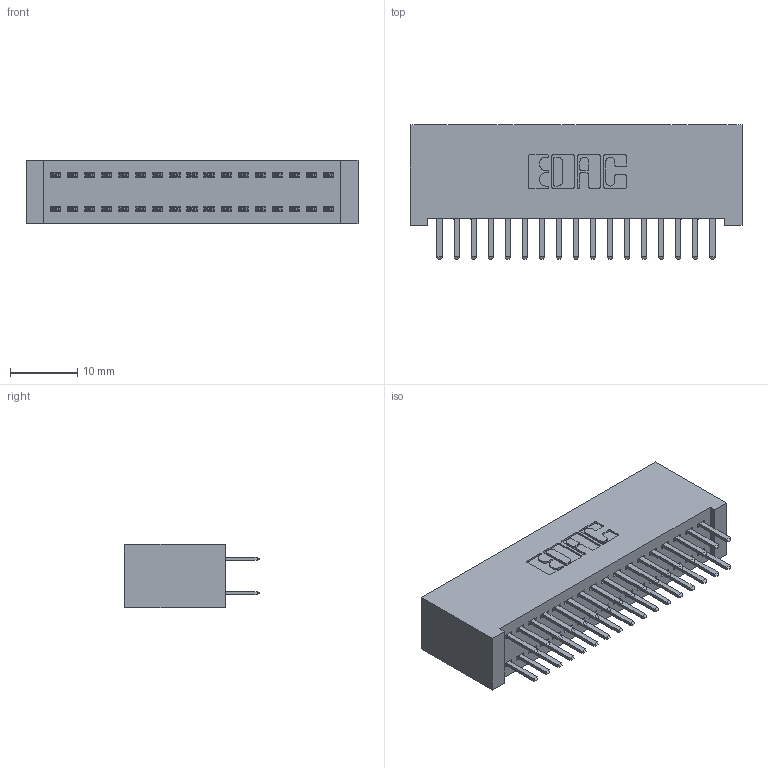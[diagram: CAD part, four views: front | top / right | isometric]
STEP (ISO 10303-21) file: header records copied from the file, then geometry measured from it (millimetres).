
FILE_DESCRIPTION (( 'STEP AP203' ), '1' );
FILE_NAME ('342-034-520-201.STEP', '2018-08-11T18:10:16', ( '' ), ( '' ), 'SwSTEP 2.0', 'SolidWorks 2016', '' );
FILE_SCHEMA (( 'CONFIG_CONTROL_DESIGN' ));
Length unit declared in the file: inch
Products named in the file (3): 342 Part_Lugless; 345-292-001_345-293-120; 342-034-520-201
Assembly tree (35 placements, depth 2):
  342-034-520-201
    342 Part_Lugless
    345-292-001_345-293-120  x34
Bounding box: 49.43 x 20.02 x 9.4 mm (x, y, z)
Volume: 4747.4 mm3; surface area: 7522.5 mm2
Topology: 35 solids, 35 shells, 2006 faces, 5817 edges, 3786 vertices
Faces by surface type: plane 1354, cylinder 652
Entity records: 13875 total; most frequent: CARTESIAN_POINT 2338, ORIENTED_EDGE 2262, DIRECTION 2023, EDGE_CURVE 1131, VECTOR 1007, LINE 1007, VERTEX_POINT 750, AXIS2_PLACEMENT_3D 508
